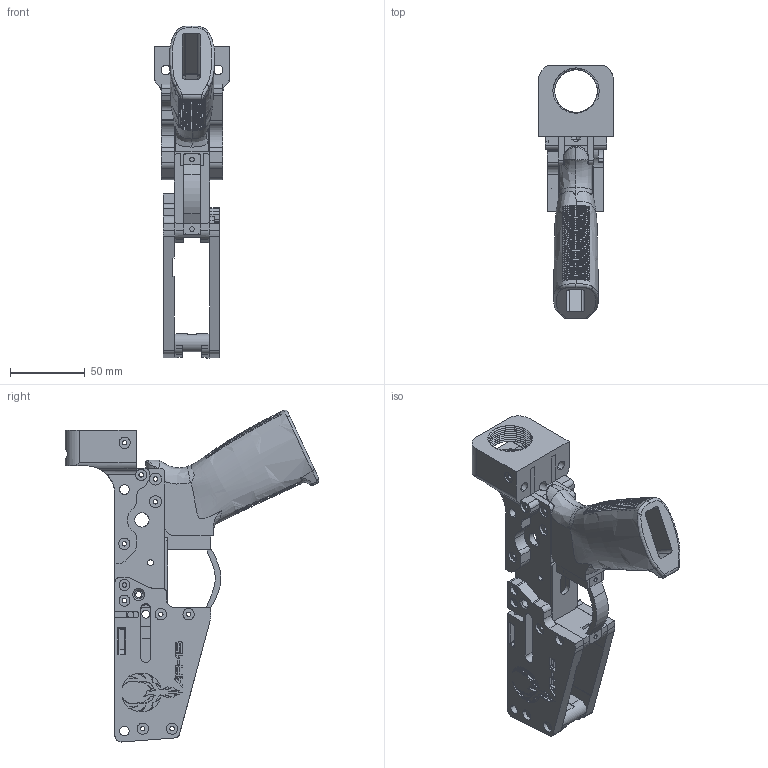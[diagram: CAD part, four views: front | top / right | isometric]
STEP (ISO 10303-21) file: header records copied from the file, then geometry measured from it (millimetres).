
FILE_DESCRIPTION (( 'STEP AP214' ), '1' );
FILE_NAME ('Firebolt_5.56_UBolt_Bolt_Catch.STEP', '2020-12-05T18:47:20', ( '' ), ( '' ), 'SwSTEP 2.0', 'SolidWorks 2020', '' );
FILE_SCHEMA (( 'AUTOMOTIVE_DESIGN' ));
Length unit declared in the file: millimetre
Products named in the file (12): Firebolt_Bolt_Catch_Mag_Well_Rear; Firebolt_Bolt_Catch_Mag_Well_Right; Firebolt_UBolt_Grip_Part; Firebolt_Fire_Control_Well_Bottom; Firebolt_UBolt_Pistol_Grip; Firebolt_Mag_Well_Front; Firebolt_Bolt_Catch_Mag_Well_Left; Firebolt_UBolt_Side_Left; Firebolt_UBolt_Buffer_Tower; Firebolt_5.56_UBolt_Bolt_Catch; Firebolt_Trigger_Guard; Firebolt_UBolt_Side_Right
Assembly tree (11 placements, depth 2):
  Firebolt_5.56_UBolt_Bolt_Catch
    Firebolt_UBolt_Buffer_Tower
    Firebolt_UBolt_Side_Left
    Firebolt_UBolt_Side_Right
    Firebolt_UBolt_Grip_Part
    Firebolt_UBolt_Pistol_Grip
    Firebolt_Fire_Control_Well_Bottom
    Firebolt_Trigger_Guard
    Firebolt_Mag_Well_Front
    Firebolt_Bolt_Catch_Mag_Well_Rear
    Firebolt_Bolt_Catch_Mag_Well_Left
    Firebolt_Bolt_Catch_Mag_Well_Right
Bounding box: 50 x 170.14 x 222.59 mm (x, y, z)
Volume: 266456.7 mm3; surface area: 120290.7 mm2
Topology: 11 solids, 11 shells, 2188 faces, 6636 edges, 4508 vertices
Faces by surface type: plane 1476, cylinder 431, bspline 265, sphere 7, cone 5, torus 4
Entity records: 139961 total; most frequent: CARTESIAN_POINT 83132, ORIENTED_EDGE 13268, DIRECTION 9490, EDGE_CURVE 6634, VERTEX_POINT 4508, VECTOR 4156, LINE 4156, AXIS2_PLACEMENT_3D 2667
